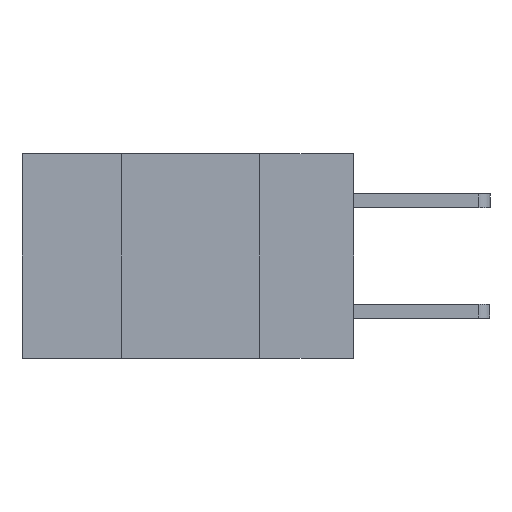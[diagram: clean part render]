
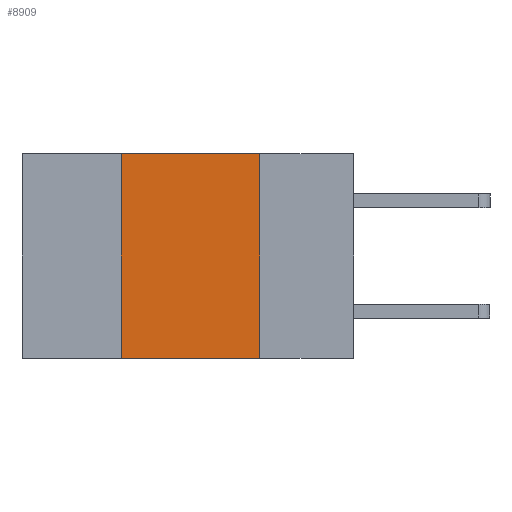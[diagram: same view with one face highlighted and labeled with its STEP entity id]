
A CAD part, left-side view. The second image highlights one B-rep face of the part: STEP entity #8909.
In plain terms, the highlighted planar face has unit normal (-1, 0, 0).
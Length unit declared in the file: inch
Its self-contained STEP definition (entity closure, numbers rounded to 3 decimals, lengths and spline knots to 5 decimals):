
#232 = VERTEX_POINT ( 'NONE', #6071 ) ;
#422 = ORIENTED_EDGE ( 'NONE', *, *, #4457, .T. ) ;
#525 = VECTOR ( 'NONE', #1056, 39.37008 ) ;
#1056 = DIRECTION ( 'NONE',  ( 0., -1., 0. ) ) ;
#1377 = ORIENTED_EDGE ( 'NONE', *, *, #10115, .F. ) ;
#1556 = PLANE ( 'NONE',  #5457 ) ;
#1890 = CARTESIAN_POINT ( 'NONE',  ( 0., 0.6, 0. ) ) ;
#2106 = VERTEX_POINT ( 'NONE', #8988 ) ;
#2159 = ORIENTED_EDGE ( 'NONE', *, *, #10011, .F. ) ;
#2915 = DIRECTION ( 'NONE',  ( 0., 0., -1. ) ) ;
#4457 = EDGE_CURVE ( 'NONE', #8020, #7077, #8793, .T. ) ;
#4549 = DIRECTION ( 'NONE',  ( 0., -1., 0. ) ) ;
#4634 = CARTESIAN_POINT ( 'NONE',  ( 0., 0.17, -0.37 ) ) ;
#4720 = DIRECTION ( 'NONE',  ( 0., 0., 1. ) ) ;
#4794 = FACE_OUTER_BOUND ( 'NONE', #10046, .T. ) ;
#5452 = LINE ( 'NONE', #9534, #9592 ) ;
#5457 = AXIS2_PLACEMENT_3D ( 'NONE', #6350, #8779, #9511 ) ;
#5912 = CARTESIAN_POINT ( 'NONE',  ( 0., 0.17, 0. ) ) ;
#6071 = CARTESIAN_POINT ( 'NONE',  ( 0., 0.42, 0. ) ) ;
#6215 = LINE ( 'NONE', #5912, #8611 ) ;
#6350 = CARTESIAN_POINT ( 'NONE',  ( 0., 0.6, 0. ) ) ;
#7077 = VERTEX_POINT ( 'NONE', #4634 ) ;
#7631 = ORIENTED_EDGE ( 'NONE', *, *, #9798, .F. ) ;
#7703 = LINE ( 'NONE', #1890, #8948 ) ;
#8020 = VERTEX_POINT ( 'NONE', #9868 ) ;
#8611 = VECTOR ( 'NONE', #2915, 39.37008 ) ;
#8779 = DIRECTION ( 'NONE',  ( 1., 0., 0. ) ) ;
#8793 = LINE ( 'NONE', #8840, #525 ) ;
#8840 = CARTESIAN_POINT ( 'NONE',  ( 0., 0.6, -0.37 ) ) ;
#8909 = ADVANCED_FACE ( 'NONE', ( #4794 ), #1556, .F. ) ;
#8948 = VECTOR ( 'NONE', #4549, 39.37008 ) ;
#8988 = CARTESIAN_POINT ( 'NONE',  ( 0., 0.17, 0. ) ) ;
#9511 = DIRECTION ( 'NONE',  ( 0., 0., -1. ) ) ;
#9534 = CARTESIAN_POINT ( 'NONE',  ( 0., 0.42, 0. ) ) ;
#9592 = VECTOR ( 'NONE', #4720, 39.37008 ) ;
#9798 = EDGE_CURVE ( 'NONE', #8020, #232, #5452, .T. ) ;
#9868 = CARTESIAN_POINT ( 'NONE',  ( 0., 0.42, -0.37 ) ) ;
#10011 = EDGE_CURVE ( 'NONE', #2106, #7077, #6215, .T. ) ;
#10046 = EDGE_LOOP ( 'NONE', ( #2159, #1377, #7631, #422 ) ) ;
#10115 = EDGE_CURVE ( 'NONE', #232, #2106, #7703, .T. ) ;
